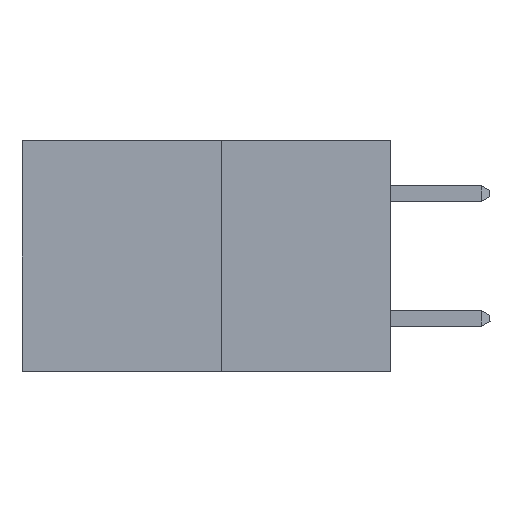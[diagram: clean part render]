
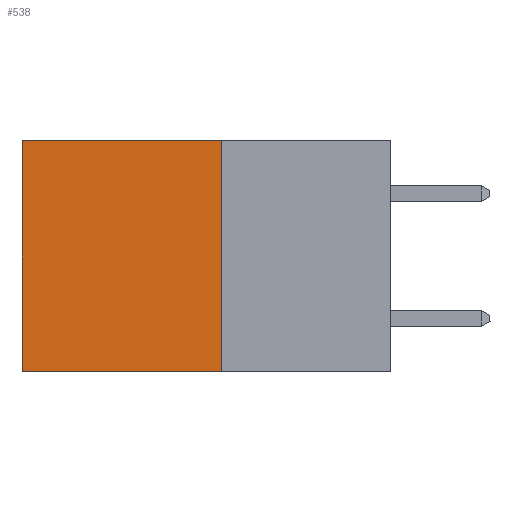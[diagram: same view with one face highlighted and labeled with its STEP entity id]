
A CAD part, left-side view. The second image highlights one B-rep face of the part: STEP entity #538.
In plain terms, the highlighted planar face has unit normal (-1, 0, 0).
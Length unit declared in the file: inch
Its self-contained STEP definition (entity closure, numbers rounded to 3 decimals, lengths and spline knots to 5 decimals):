
#291 = CARTESIAN_POINT ( 'NONE',  ( 0.277, 0.59, -0.37 ) ) ;
#538 = ADVANCED_FACE ( 'NONE', ( #15768 ), #5222, .F. ) ;
#934 = EDGE_CURVE ( 'NONE', #12739, #14504, #9575, .T. ) ;
#1432 = CARTESIAN_POINT ( 'NONE',  ( 0.277, 0.27, -0.37 ) ) ;
#2348 = VECTOR ( 'NONE', #9806, 39.37008 ) ;
#2563 = ORIENTED_EDGE ( 'NONE', *, *, #8043, .F. ) ;
#3965 = VERTEX_POINT ( 'NONE', #15435 ) ;
#4922 = CARTESIAN_POINT ( 'NONE',  ( 0.277, 0.59, 0. ) ) ;
#5222 = PLANE ( 'NONE',  #7026 ) ;
#5325 = DIRECTION ( 'NONE',  ( 0., 1., 0. ) ) ;
#5950 = VECTOR ( 'NONE', #9608, 39.37008 ) ;
#6398 = EDGE_LOOP ( 'NONE', ( #6908, #16002, #2563, #6415 ) ) ;
#6415 = ORIENTED_EDGE ( 'NONE', *, *, #934, .T. ) ;
#6908 = ORIENTED_EDGE ( 'NONE', *, *, #7598, .T. ) ;
#7026 = AXIS2_PLACEMENT_3D ( 'NONE', #7881, #15536, #15540 ) ;
#7598 = EDGE_CURVE ( 'NONE', #14504, #3965, #16078, .T. ) ;
#7881 = CARTESIAN_POINT ( 'NONE',  ( 0.277, 0.27, -0.37 ) ) ;
#8043 = EDGE_CURVE ( 'NONE', #12739, #12104, #16475, .T. ) ;
#8993 = EDGE_CURVE ( 'NONE', #12104, #3965, #9023, .T. ) ;
#9023 = LINE ( 'NONE', #16366, #2348 ) ;
#9328 = CARTESIAN_POINT ( 'NONE',  ( 0.277, 0.27, 0. ) ) ;
#9575 = LINE ( 'NONE', #9711, #16160 ) ;
#9608 = DIRECTION ( 'NONE',  ( 0., 0., -1. ) ) ;
#9711 = CARTESIAN_POINT ( 'NONE',  ( 0.277, 0.27, 0. ) ) ;
#9806 = DIRECTION ( 'NONE',  ( 0., 1., 0. ) ) ;
#12104 = VERTEX_POINT ( 'NONE', #1432 ) ;
#12739 = VERTEX_POINT ( 'NONE', #9328 ) ;
#13029 = VECTOR ( 'NONE', #16971, 39.37008 ) ;
#13039 = CARTESIAN_POINT ( 'NONE',  ( 0.277, 0.27, -0.37 ) ) ;
#14504 = VERTEX_POINT ( 'NONE', #4922 ) ;
#15435 = CARTESIAN_POINT ( 'NONE',  ( 0.277, 0.59, -0.37 ) ) ;
#15536 = DIRECTION ( 'NONE',  ( 1., 0., 0. ) ) ;
#15540 = DIRECTION ( 'NONE',  ( 0., 0., -1. ) ) ;
#15768 = FACE_OUTER_BOUND ( 'NONE', #6398, .T. ) ;
#16002 = ORIENTED_EDGE ( 'NONE', *, *, #8993, .F. ) ;
#16078 = LINE ( 'NONE', #291, #5950 ) ;
#16160 = VECTOR ( 'NONE', #5325, 39.37008 ) ;
#16366 = CARTESIAN_POINT ( 'NONE',  ( 0.277, 0.27, -0.37 ) ) ;
#16475 = LINE ( 'NONE', #13039, #13029 ) ;
#16971 = DIRECTION ( 'NONE',  ( 0., 0., -1. ) ) ;
